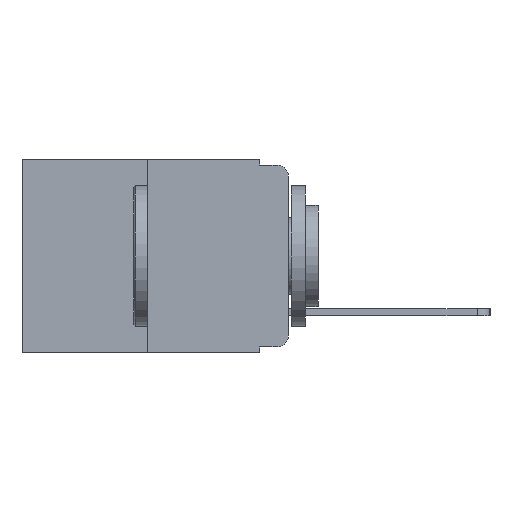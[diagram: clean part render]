
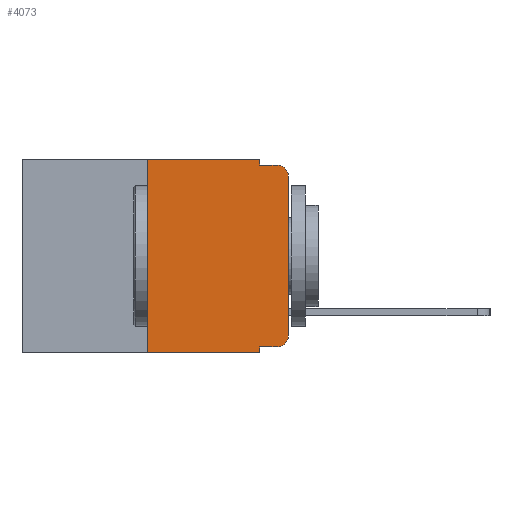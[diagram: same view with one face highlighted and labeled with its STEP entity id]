
A CAD part, left-side view. The second image highlights one B-rep face of the part: STEP entity #4073.
In plain terms, the highlighted planar face has unit normal (-1, 0, 0).
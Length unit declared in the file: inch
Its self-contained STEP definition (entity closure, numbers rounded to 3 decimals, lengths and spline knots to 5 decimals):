
#356 = VECTOR ( 'NONE', #11115, 39.37008 ) ;
#681 = ORIENTED_EDGE ( 'NONE', *, *, #11812, .F. ) ;
#908 = VERTEX_POINT ( 'NONE', #4944 ) ;
#926 = DIRECTION ( 'NONE',  ( 0., 0., -1. ) ) ;
#1206 = EDGE_CURVE ( 'NONE', #1494, #4707, #8047, .T. ) ;
#1418 = CARTESIAN_POINT ( 'NONE',  ( 0., 0.473, 0. ) ) ;
#1494 = VERTEX_POINT ( 'NONE', #5412 ) ;
#1588 = EDGE_CURVE ( 'NONE', #4707, #5031, #11316, .T. ) ;
#1721 = CARTESIAN_POINT ( 'NONE',  ( 0., 0., -0.313 ) ) ;
#1855 = ORIENTED_EDGE ( 'NONE', *, *, #9572, .F. ) ;
#1930 = AXIS2_PLACEMENT_3D ( 'NONE', #1418, #5008, #4994 ) ;
#2024 = LINE ( 'NONE', #3566, #4864 ) ;
#2383 = CARTESIAN_POINT ( 'NONE',  ( 0., 0.051, 0. ) ) ;
#2923 = LINE ( 'NONE', #5346, #10294 ) ;
#2939 = VECTOR ( 'NONE', #11221, 39.37008 ) ;
#2956 = VERTEX_POINT ( 'NONE', #13026 ) ;
#2958 = DIRECTION ( 'NONE',  ( 0., 0., -1. ) ) ;
#2968 = ORIENTED_EDGE ( 'NONE', *, *, #1206, .T. ) ;
#3225 = ORIENTED_EDGE ( 'NONE', *, *, #13756, .F. ) ;
#3403 = PLANE ( 'NONE',  #1930 ) ;
#3499 = EDGE_CURVE ( 'NONE', #5031, #908, #4828, .T. ) ;
#3566 = CARTESIAN_POINT ( 'NONE',  ( 0., 0.051, 0. ) ) ;
#3594 = VERTEX_POINT ( 'NONE', #9218 ) ;
#3626 = CARTESIAN_POINT ( 'NONE',  ( 0., 0.051, -0.333 ) ) ;
#3800 = DIRECTION ( 'NONE',  ( 0., -1., 0. ) ) ;
#4073 = ADVANCED_FACE ( 'NONE', ( #10053 ), #3403, .F. ) ;
#4707 = VERTEX_POINT ( 'NONE', #1721 ) ;
#4828 = CIRCLE ( 'NONE', #10250, 0.02 ) ;
#4864 = VECTOR ( 'NONE', #926, 39.37008 ) ;
#4944 = CARTESIAN_POINT ( 'NONE',  ( 0., 0.02, -0.01 ) ) ;
#4994 = DIRECTION ( 'NONE',  ( 0., 0., -1. ) ) ;
#5008 = DIRECTION ( 'NONE',  ( 1., 0., 0. ) ) ;
#5031 = VERTEX_POINT ( 'NONE', #11030 ) ;
#5292 = VECTOR ( 'NONE', #11329, 39.37008 ) ;
#5335 = CARTESIAN_POINT ( 'NONE',  ( 0., 0.051, -0.343 ) ) ;
#5346 = CARTESIAN_POINT ( 'NONE',  ( 0., 0.25, 0. ) ) ;
#5412 = CARTESIAN_POINT ( 'NONE',  ( 0., 0.02, -0.333 ) ) ;
#5922 = VERTEX_POINT ( 'NONE', #13575 ) ;
#6032 = LINE ( 'NONE', #3626, #2939 ) ;
#6051 = EDGE_CURVE ( 'NONE', #5922, #1494, #6032, .T. ) ;
#6311 = VERTEX_POINT ( 'NONE', #5335 ) ;
#6756 = ORIENTED_EDGE ( 'NONE', *, *, #6051, .T. ) ;
#7084 = CARTESIAN_POINT ( 'NONE',  ( 0., 0.02, -0.03 ) ) ;
#7151 = EDGE_LOOP ( 'NONE', ( #9168, #13400, #9874, #1855, #3225, #681, #12156, #7609, #6756, #2968 ) ) ;
#7609 = ORIENTED_EDGE ( 'NONE', *, *, #10838, .F. ) ;
#7709 = EDGE_CURVE ( 'NONE', #3594, #908, #13995, .T. ) ;
#8047 = CIRCLE ( 'NONE', #12761, 0.02 ) ;
#8068 = CARTESIAN_POINT ( 'NONE',  ( 0., 0.051, 0. ) ) ;
#8297 = VERTEX_POINT ( 'NONE', #8068 ) ;
#8337 = VECTOR ( 'NONE', #12383, 39.37008 ) ;
#8893 = CARTESIAN_POINT ( 'NONE',  ( 0., 0.473, -0.343 ) ) ;
#9168 = ORIENTED_EDGE ( 'NONE', *, *, #1588, .T. ) ;
#9218 = CARTESIAN_POINT ( 'NONE',  ( 0., 0.051, -0.01 ) ) ;
#9311 = CARTESIAN_POINT ( 'NONE',  ( 0., 0.473, 0. ) ) ;
#9440 = DIRECTION ( 'NONE',  ( 0., 0., -1. ) ) ;
#9463 = LINE ( 'NONE', #9311, #11751 ) ;
#9572 = EDGE_CURVE ( 'NONE', #8297, #3594, #9954, .T. ) ;
#9754 = DIRECTION ( 'NONE',  ( -1., 0., 0. ) ) ;
#9874 = ORIENTED_EDGE ( 'NONE', *, *, #7709, .F. ) ;
#9930 = DIRECTION ( 'NONE',  ( 0., -1., 0. ) ) ;
#9954 = LINE ( 'NONE', #2383, #356 ) ;
#10053 = FACE_OUTER_BOUND ( 'NONE', #7151, .T. ) ;
#10246 = LINE ( 'NONE', #8893, #12510 ) ;
#10250 = AXIS2_PLACEMENT_3D ( 'NONE', #7084, #9754, #9440 ) ;
#10294 = VECTOR ( 'NONE', #13487, 39.37008 ) ;
#10838 = EDGE_CURVE ( 'NONE', #5922, #6311, #2024, .T. ) ;
#11030 = CARTESIAN_POINT ( 'NONE',  ( 0., 0., -0.03 ) ) ;
#11115 = DIRECTION ( 'NONE',  ( 0., 0., -1. ) ) ;
#11221 = DIRECTION ( 'NONE',  ( 0., -1., 0. ) ) ;
#11316 = LINE ( 'NONE', #12163, #8337 ) ;
#11329 = DIRECTION ( 'NONE',  ( 0., -1., 0. ) ) ;
#11751 = VECTOR ( 'NONE', #3800, 39.37008 ) ;
#11812 = EDGE_CURVE ( 'NONE', #13255, #2956, #2923, .T. ) ;
#12156 = ORIENTED_EDGE ( 'NONE', *, *, #13449, .T. ) ;
#12163 = CARTESIAN_POINT ( 'NONE',  ( 0., 0., 0. ) ) ;
#12383 = DIRECTION ( 'NONE',  ( 0., 0., 1. ) ) ;
#12510 = VECTOR ( 'NONE', #9930, 39.37008 ) ;
#12761 = AXIS2_PLACEMENT_3D ( 'NONE', #13313, #13261, #2958 ) ;
#13026 = CARTESIAN_POINT ( 'NONE',  ( 0., 0.25, 0. ) ) ;
#13207 = CARTESIAN_POINT ( 'NONE',  ( 0., 0.051, -0.01 ) ) ;
#13255 = VERTEX_POINT ( 'NONE', #13457 ) ;
#13261 = DIRECTION ( 'NONE',  ( -1., 0., 0. ) ) ;
#13313 = CARTESIAN_POINT ( 'NONE',  ( 0., 0.02, -0.313 ) ) ;
#13400 = ORIENTED_EDGE ( 'NONE', *, *, #3499, .T. ) ;
#13449 = EDGE_CURVE ( 'NONE', #13255, #6311, #10246, .T. ) ;
#13457 = CARTESIAN_POINT ( 'NONE',  ( 0., 0.25, -0.343 ) ) ;
#13487 = DIRECTION ( 'NONE',  ( 0., 0., 1. ) ) ;
#13575 = CARTESIAN_POINT ( 'NONE',  ( 0., 0.051, -0.333 ) ) ;
#13756 = EDGE_CURVE ( 'NONE', #2956, #8297, #9463, .T. ) ;
#13995 = LINE ( 'NONE', #13207, #5292 ) ;
